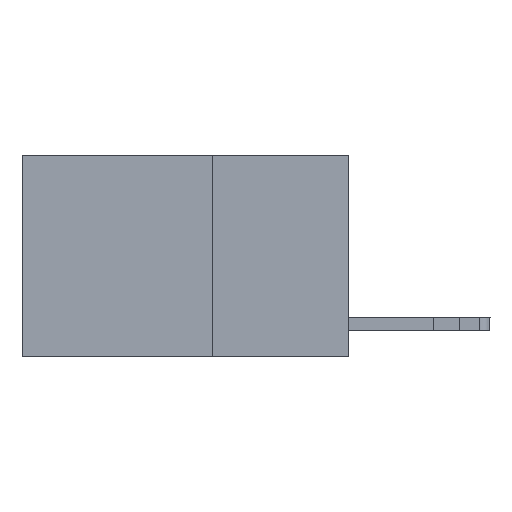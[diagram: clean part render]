
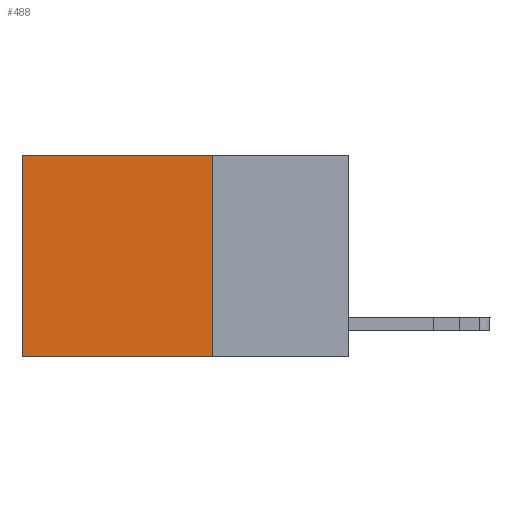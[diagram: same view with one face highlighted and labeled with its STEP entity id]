
A CAD part, left-side view. The second image highlights one B-rep face of the part: STEP entity #488.
In plain terms, the highlighted planar face has unit normal (-1, 0, 0).
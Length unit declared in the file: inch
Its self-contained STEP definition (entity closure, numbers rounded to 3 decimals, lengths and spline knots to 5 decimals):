
#289 = CARTESIAN_POINT ( 'NONE',  ( 0.2625, 0.25, 0. ) ) ;
#488 = ADVANCED_FACE ( 'NONE', ( #11230 ), #2173, .F. ) ;
#643 = VERTEX_POINT ( 'NONE', #974 ) ;
#743 = CARTESIAN_POINT ( 'NONE',  ( 0.2625, 0.25, 0. ) ) ;
#926 = AXIS2_PLACEMENT_3D ( 'NONE', #743, #11693, #7040 ) ;
#974 = CARTESIAN_POINT ( 'NONE',  ( 0.2625, 0.25, 0. ) ) ;
#1650 = LINE ( 'NONE', #5622, #16106 ) ;
#2173 = PLANE ( 'NONE',  #926 ) ;
#2245 = EDGE_CURVE ( 'NONE', #643, #19134, #6808, .T. ) ;
#3641 = ORIENTED_EDGE ( 'NONE', *, *, #9404, .T. ) ;
#4754 = VERTEX_POINT ( 'NONE', #20057 ) ;
#5622 = CARTESIAN_POINT ( 'NONE',  ( 0.2625, 0.6, 0. ) ) ;
#6131 = CARTESIAN_POINT ( 'NONE',  ( 0.2625, 0.25, -0.37 ) ) ;
#6808 = LINE ( 'NONE', #14797, #20149 ) ;
#7040 = DIRECTION ( 'NONE',  ( 0., 0., -1. ) ) ;
#7359 = DIRECTION ( 'NONE',  ( 0., 0., -1. ) ) ;
#8205 = CARTESIAN_POINT ( 'NONE',  ( 0.2625, 0.25, -0.37 ) ) ;
#8879 = ORIENTED_EDGE ( 'NONE', *, *, #14925, .T. ) ;
#9054 = VECTOR ( 'NONE', #17780, 39.37008 ) ;
#9404 = EDGE_CURVE ( 'NONE', #643, #4754, #9607, .T. ) ;
#9607 = LINE ( 'NONE', #289, #9054 ) ;
#11230 = FACE_OUTER_BOUND ( 'NONE', #17231, .T. ) ;
#11693 = DIRECTION ( 'NONE',  ( 1., 0., 0. ) ) ;
#12302 = EDGE_CURVE ( 'NONE', #19134, #21634, #21961, .T. ) ;
#13067 = DIRECTION ( 'NONE',  ( 0., 0., -1. ) ) ;
#13406 = ORIENTED_EDGE ( 'NONE', *, *, #12302, .F. ) ;
#14797 = CARTESIAN_POINT ( 'NONE',  ( 0.2625, 0.25, 0. ) ) ;
#14925 = EDGE_CURVE ( 'NONE', #4754, #21634, #1650, .T. ) ;
#16106 = VECTOR ( 'NONE', #7359, 39.37008 ) ;
#17231 = EDGE_LOOP ( 'NONE', ( #8879, #13406, #18578, #3641 ) ) ;
#17780 = DIRECTION ( 'NONE',  ( 0., 1., 0. ) ) ;
#18578 = ORIENTED_EDGE ( 'NONE', *, *, #2245, .F. ) ;
#19134 = VERTEX_POINT ( 'NONE', #8205 ) ;
#20057 = CARTESIAN_POINT ( 'NONE',  ( 0.2625, 0.6, 0. ) ) ;
#20149 = VECTOR ( 'NONE', #13067, 39.37008 ) ;
#21425 = VECTOR ( 'NONE', #21792, 39.37008 ) ;
#21634 = VERTEX_POINT ( 'NONE', #21919 ) ;
#21792 = DIRECTION ( 'NONE',  ( 0., 1., 0. ) ) ;
#21919 = CARTESIAN_POINT ( 'NONE',  ( 0.2625, 0.6, -0.37 ) ) ;
#21961 = LINE ( 'NONE', #6131, #21425 ) ;
